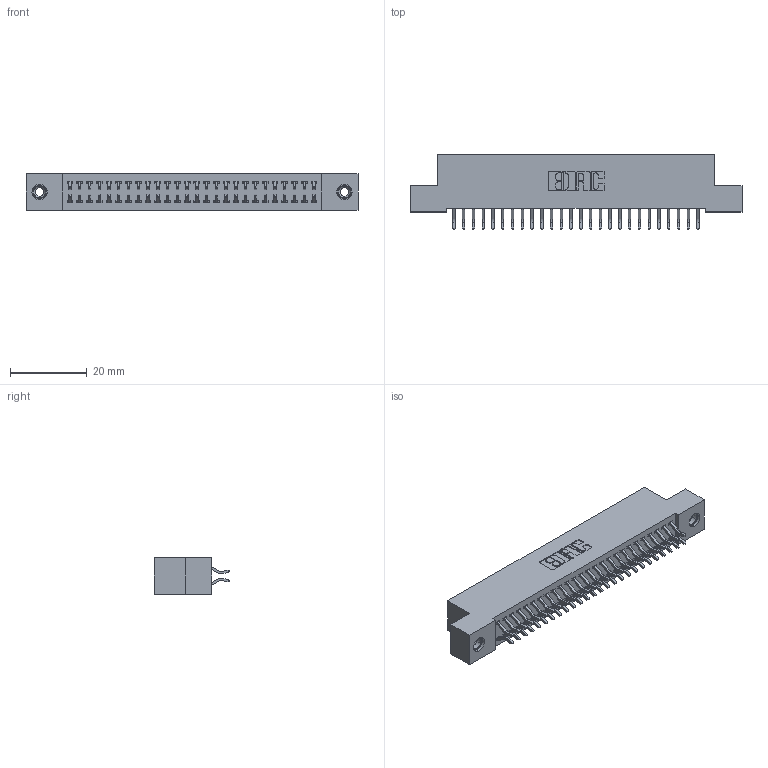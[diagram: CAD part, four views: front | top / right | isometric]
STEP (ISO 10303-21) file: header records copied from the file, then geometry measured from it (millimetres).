
FILE_DESCRIPTION (( 'STEP AP203' ), '1' );
FILE_NAME ('392-052-556-208.STEP', '2018-08-17T06:15:41', ( '' ), ( '' ), 'SwSTEP 2.0', 'SolidWorks 2016', '' );
FILE_SCHEMA (( 'CONFIG_CONTROL_DESIGN' ));
Length unit declared in the file: inch
Products named in the file (4): 342 Part_TI; 345-292-001_556 Tail; 345-250-001_345-250-003-102; 392-052-556-208
Assembly tree (55 placements, depth 2):
  392-052-556-208
    342 Part_TI
    345-292-001_556 Tail  x52
    345-250-001_345-250-003-102  x2
Bounding box: 86.36 x 19.58 x 9.4 mm (x, y, z)
Volume: 7676.7 mm3; surface area: 12061.3 mm2
Topology: 55 solids, 55 shells, 3186 faces, 9431 edges, 6210 vertices
Faces by surface type: plane 2178, cylinder 992, cone 12, torus 4
Entity records: 20070 total; most frequent: CARTESIAN_POINT 3341, ORIENTED_EDGE 3258, DIRECTION 2903, EDGE_CURVE 1629, LINE 1473, VECTOR 1473, VERTEX_POINT 1080, AXIS2_PLACEMENT_3D 715
